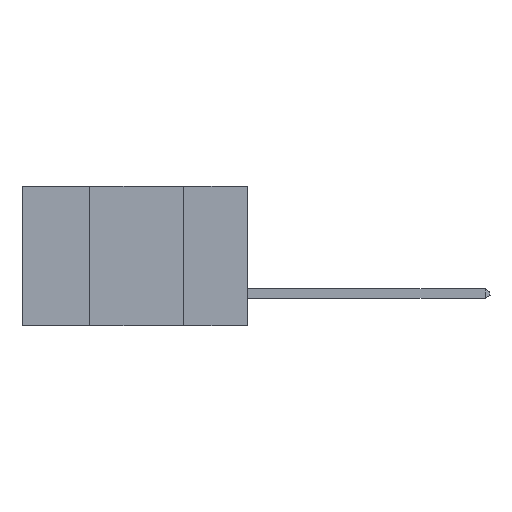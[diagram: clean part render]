
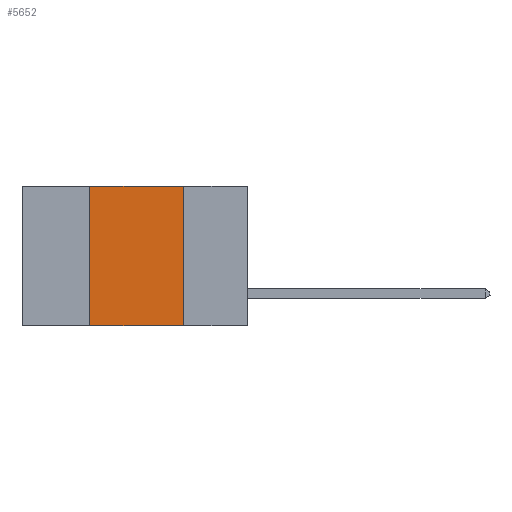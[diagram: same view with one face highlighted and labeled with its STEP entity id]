
A CAD part, left-side view. The second image highlights one B-rep face of the part: STEP entity #5652.
In plain terms, the highlighted planar face has unit normal (-1, 0, 0).
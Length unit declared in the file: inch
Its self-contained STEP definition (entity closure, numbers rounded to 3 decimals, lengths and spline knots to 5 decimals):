
#462 = VECTOR ( 'NONE', #5084, 39.37008 ) ;
#609 = CARTESIAN_POINT ( 'NONE',  ( 0., 0.42, 0. ) ) ;
#621 = LINE ( 'NONE', #609, #2023 ) ;
#1848 = DIRECTION ( 'NONE',  ( 1., 0., 0. ) ) ;
#1964 = CARTESIAN_POINT ( 'NONE',  ( 0., 0.17, 0. ) ) ;
#2004 = VERTEX_POINT ( 'NONE', #17764 ) ;
#2023 = VECTOR ( 'NONE', #5761, 39.37008 ) ;
#2173 = VERTEX_POINT ( 'NONE', #7968 ) ;
#2351 = FACE_OUTER_BOUND ( 'NONE', #5260, .T. ) ;
#2657 = CARTESIAN_POINT ( 'NONE',  ( 0., 0.6, -0.37 ) ) ;
#3394 = DIRECTION ( 'NONE',  ( 0., -1., 0. ) ) ;
#3572 = CARTESIAN_POINT ( 'NONE',  ( 0., 0.42, 0. ) ) ;
#3992 = ORIENTED_EDGE ( 'NONE', *, *, #5918, .F. ) ;
#5084 = DIRECTION ( 'NONE',  ( 0., 0., -1. ) ) ;
#5110 = VERTEX_POINT ( 'NONE', #3572 ) ;
#5260 = EDGE_LOOP ( 'NONE', ( #3992, #13323, #12054, #11890 ) ) ;
#5652 = ADVANCED_FACE ( 'NONE', ( #2351 ), #7924, .F. ) ;
#5761 = DIRECTION ( 'NONE',  ( 0., 0., 1. ) ) ;
#5918 = EDGE_CURVE ( 'NONE', #7872, #2173, #17608, .T. ) ;
#6200 = VECTOR ( 'NONE', #14820, 39.37008 ) ;
#7585 = EDGE_CURVE ( 'NONE', #2004, #5110, #621, .T. ) ;
#7872 = VERTEX_POINT ( 'NONE', #1964 ) ;
#7924 = PLANE ( 'NONE',  #15951 ) ;
#7968 = CARTESIAN_POINT ( 'NONE',  ( 0., 0.17, -0.37 ) ) ;
#8139 = CARTESIAN_POINT ( 'NONE',  ( 0., 0.6, 0. ) ) ;
#9120 = LINE ( 'NONE', #18736, #16297 ) ;
#9225 = EDGE_CURVE ( 'NONE', #5110, #7872, #9120, .T. ) ;
#9638 = CARTESIAN_POINT ( 'NONE',  ( 0., 0.17, 0. ) ) ;
#11890 = ORIENTED_EDGE ( 'NONE', *, *, #13854, .T. ) ;
#12054 = ORIENTED_EDGE ( 'NONE', *, *, #7585, .F. ) ;
#13323 = ORIENTED_EDGE ( 'NONE', *, *, #9225, .F. ) ;
#13854 = EDGE_CURVE ( 'NONE', #2004, #2173, #14323, .T. ) ;
#14323 = LINE ( 'NONE', #2657, #6200 ) ;
#14820 = DIRECTION ( 'NONE',  ( 0., -1., 0. ) ) ;
#15951 = AXIS2_PLACEMENT_3D ( 'NONE', #8139, #1848, #18785 ) ;
#16297 = VECTOR ( 'NONE', #3394, 39.37008 ) ;
#17608 = LINE ( 'NONE', #9638, #462 ) ;
#17764 = CARTESIAN_POINT ( 'NONE',  ( 0., 0.42, -0.37 ) ) ;
#18736 = CARTESIAN_POINT ( 'NONE',  ( 0., 0.6, 0. ) ) ;
#18785 = DIRECTION ( 'NONE',  ( 0., 0., -1. ) ) ;
